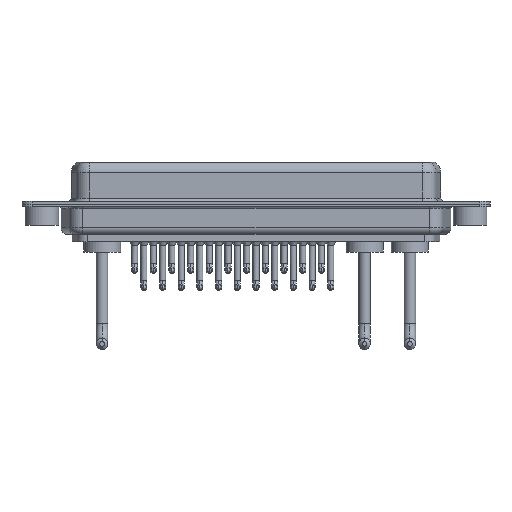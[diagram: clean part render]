
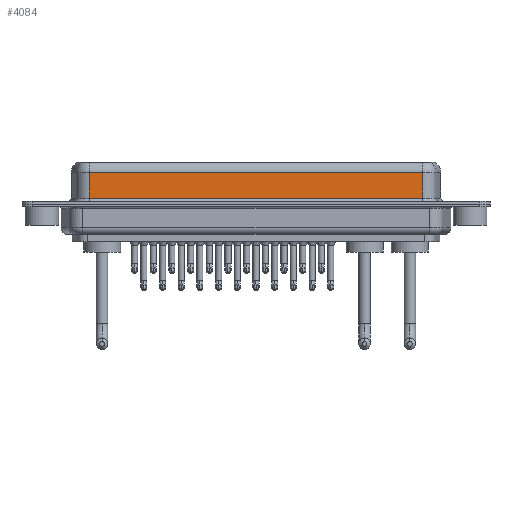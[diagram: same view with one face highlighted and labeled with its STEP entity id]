
A CAD part, front view. The second image highlights one B-rep face of the part: STEP entity #4084.
In plain terms, the highlighted planar face has unit normal (0, -1, 0).
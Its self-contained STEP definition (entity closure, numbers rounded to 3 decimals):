
#981 = VERTEX_POINT ( 'NONE', #12200 ) ;
#1203 = EDGE_CURVE ( 'NONE', #981, #18225, #18554, .T. ) ;
#1505 = LINE ( 'NONE', #19777, #23048 ) ;
#1657 = LINE ( 'NONE', #3693, #6118 ) ;
#1747 = FACE_OUTER_BOUND ( 'NONE', #13873, .T. ) ;
#1826 = VECTOR ( 'NONE', #5361, 1000. ) ;
#3693 = CARTESIAN_POINT ( 'NONE',  ( 56.462, -3.95, 6.4 ) ) ;
#4084 = ADVANCED_FACE ( 'NONE', ( #1747 ), #17971, .F. ) ;
#4582 = VERTEX_POINT ( 'NONE', #9016 ) ;
#5361 = DIRECTION ( 'NONE',  ( -1., 0., 0. ) ) ;
#6118 = VECTOR ( 'NONE', #7417, 1000. ) ;
#7376 = EDGE_CURVE ( 'NONE', #981, #13251, #1657, .T. ) ;
#7417 = DIRECTION ( 'NONE',  ( 0., 0., -1. ) ) ;
#7775 = EDGE_CURVE ( 'NONE', #18225, #4582, #1505, .T. ) ;
#9016 = CARTESIAN_POINT ( 'NONE',  ( 7.038, -3.95, 0.9 ) ) ;
#9072 = DIRECTION ( 'NONE',  ( 0., 0., 1. ) ) ;
#9311 = CARTESIAN_POINT ( 'NONE',  ( 7.038, -3.95, 4.65 ) ) ;
#10160 = DIRECTION ( 'NONE',  ( 0., 0., -1. ) ) ;
#10882 = CARTESIAN_POINT ( 'NONE',  ( 56.462, -3.95, 6.4 ) ) ;
#11707 = LINE ( 'NONE', #17121, #21096 ) ;
#11789 = ORIENTED_EDGE ( 'NONE', *, *, #1203, .T. ) ;
#12200 = CARTESIAN_POINT ( 'NONE',  ( 56.462, -3.95, 4.65 ) ) ;
#13047 = ORIENTED_EDGE ( 'NONE', *, *, #7775, .T. ) ;
#13147 = CARTESIAN_POINT ( 'NONE',  ( 56.462, -3.95, 4.65 ) ) ;
#13251 = VERTEX_POINT ( 'NONE', #13692 ) ;
#13692 = CARTESIAN_POINT ( 'NONE',  ( 56.462, -3.95, 0.9 ) ) ;
#13873 = EDGE_LOOP ( 'NONE', ( #18274, #11789, #13047, #18068 ) ) ;
#14071 = EDGE_CURVE ( 'NONE', #4582, #13251, #11707, .T. ) ;
#15412 = AXIS2_PLACEMENT_3D ( 'NONE', #10882, #16178, #9072 ) ;
#15553 = DIRECTION ( 'NONE',  ( 1., 0., 0. ) ) ;
#16178 = DIRECTION ( 'NONE',  ( 0., 1., 0. ) ) ;
#17121 = CARTESIAN_POINT ( 'NONE',  ( 56.462, -3.95, 0.9 ) ) ;
#17971 = PLANE ( 'NONE',  #15412 ) ;
#18068 = ORIENTED_EDGE ( 'NONE', *, *, #14071, .T. ) ;
#18225 = VERTEX_POINT ( 'NONE', #9311 ) ;
#18274 = ORIENTED_EDGE ( 'NONE', *, *, #7376, .F. ) ;
#18554 = LINE ( 'NONE', #13147, #1826 ) ;
#19777 = CARTESIAN_POINT ( 'NONE',  ( 7.038, -3.95, 6.4 ) ) ;
#21096 = VECTOR ( 'NONE', #15553, 1000. ) ;
#23048 = VECTOR ( 'NONE', #10160, 1000. ) ;
